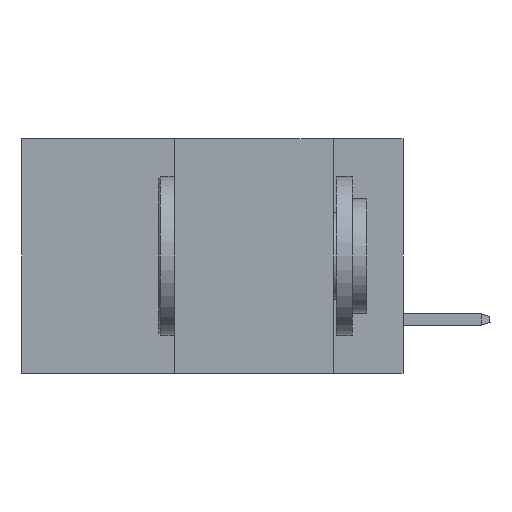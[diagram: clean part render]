
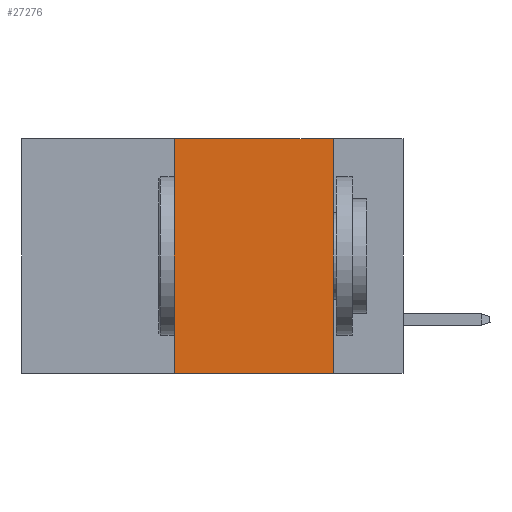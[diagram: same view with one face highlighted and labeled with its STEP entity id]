
A CAD part, left-side view. The second image highlights one B-rep face of the part: STEP entity #27276.
In plain terms, the highlighted planar face has unit normal (-1, 0, 0).
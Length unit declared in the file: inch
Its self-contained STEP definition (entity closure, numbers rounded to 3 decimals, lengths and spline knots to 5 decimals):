
#339 = ORIENTED_EDGE ( 'NONE', *, *, #24955, .T. ) ;
#2707 = DIRECTION ( 'NONE',  ( 1., 0., 0. ) ) ;
#2935 = FACE_OUTER_BOUND ( 'NONE', #31308, .T. ) ;
#3025 = VERTEX_POINT ( 'NONE', #16048 ) ;
#3089 = ORIENTED_EDGE ( 'NONE', *, *, #8750, .F. ) ;
#4392 = AXIS2_PLACEMENT_3D ( 'NONE', #28214, #2707, #19545 ) ;
#6230 = VECTOR ( 'NONE', #28458, 39.37008 ) ;
#7533 = CARTESIAN_POINT ( 'NONE',  ( 0., 0.11, 0. ) ) ;
#8750 = EDGE_CURVE ( 'NONE', #11333, #34213, #12200, .T. ) ;
#11333 = VERTEX_POINT ( 'NONE', #43247 ) ;
#11857 = VECTOR ( 'NONE', #29249, 39.37008 ) ;
#12200 = LINE ( 'NONE', #12657, #35857 ) ;
#12657 = CARTESIAN_POINT ( 'NONE',  ( 0., 0.6, 0. ) ) ;
#12930 = CARTESIAN_POINT ( 'NONE',  ( 0., 0.11, 0. ) ) ;
#13456 = LINE ( 'NONE', #42253, #15579 ) ;
#14423 = VERTEX_POINT ( 'NONE', #26515 ) ;
#15579 = VECTOR ( 'NONE', #24303, 39.37008 ) ;
#16048 = CARTESIAN_POINT ( 'NONE',  ( 0., 0.11, -0.37 ) ) ;
#19545 = DIRECTION ( 'NONE',  ( 0., 0., -1. ) ) ;
#21488 = ORIENTED_EDGE ( 'NONE', *, *, #25060, .F. ) ;
#24219 = CARTESIAN_POINT ( 'NONE',  ( 0., 0.36, 0. ) ) ;
#24303 = DIRECTION ( 'NONE',  ( 0., -1., 0. ) ) ;
#24955 = EDGE_CURVE ( 'NONE', #14423, #3025, #13456, .T. ) ;
#25060 = EDGE_CURVE ( 'NONE', #34213, #3025, #39882, .T. ) ;
#26515 = CARTESIAN_POINT ( 'NONE',  ( 0., 0.36, -0.37 ) ) ;
#27276 = ADVANCED_FACE ( 'NONE', ( #2935 ), #45698, .F. ) ;
#28214 = CARTESIAN_POINT ( 'NONE',  ( 0., 0.6, 0. ) ) ;
#28458 = DIRECTION ( 'NONE',  ( 0., 0., 1. ) ) ;
#29249 = DIRECTION ( 'NONE',  ( 0., 0., -1. ) ) ;
#29897 = DIRECTION ( 'NONE',  ( 0., -1., 0. ) ) ;
#31308 = EDGE_LOOP ( 'NONE', ( #21488, #3089, #42057, #339 ) ) ;
#34213 = VERTEX_POINT ( 'NONE', #12930 ) ;
#35857 = VECTOR ( 'NONE', #29897, 39.37008 ) ;
#35966 = EDGE_CURVE ( 'NONE', #14423, #11333, #42169, .T. ) ;
#39882 = LINE ( 'NONE', #7533, #11857 ) ;
#42057 = ORIENTED_EDGE ( 'NONE', *, *, #35966, .F. ) ;
#42169 = LINE ( 'NONE', #24219, #6230 ) ;
#42253 = CARTESIAN_POINT ( 'NONE',  ( 0., 0.6, -0.37 ) ) ;
#43247 = CARTESIAN_POINT ( 'NONE',  ( 0., 0.36, 0. ) ) ;
#45698 = PLANE ( 'NONE',  #4392 ) ;
